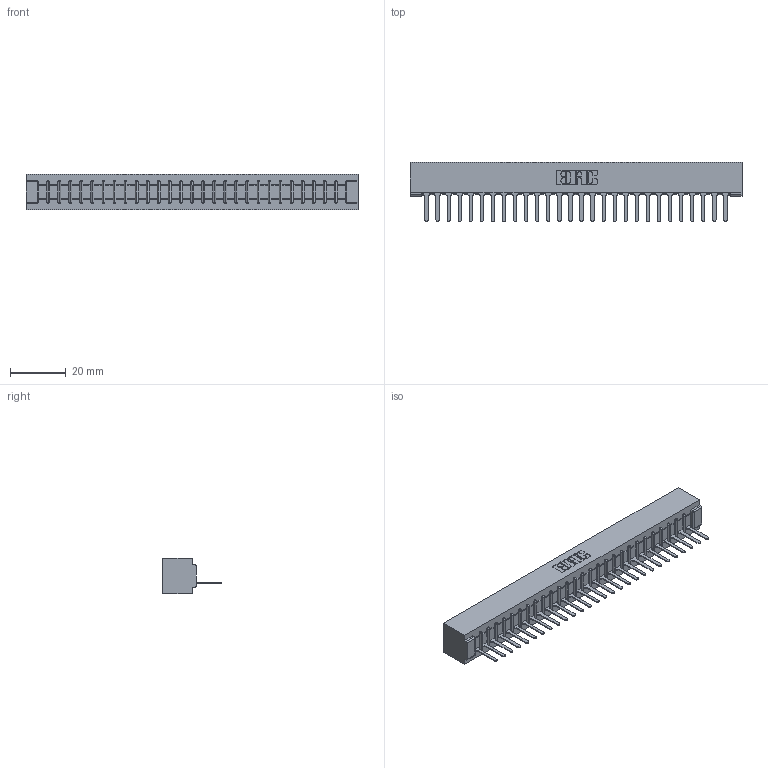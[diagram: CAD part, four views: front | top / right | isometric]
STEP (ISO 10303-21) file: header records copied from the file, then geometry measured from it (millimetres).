
FILE_DESCRIPTION (( 'STEP AP203' ), '1' );
FILE_NAME ('357-028-427-101.STEP', '2020-10-01T20:28:08', ( '' ), ( '' ), 'SwSTEP 2.0', 'SolidWorks 2020', '' );
FILE_SCHEMA (( 'CONFIG_CONTROL_DESIGN' ));
Length unit declared in the file: inch
Products named in the file (3): 307-290-001_527; 307 Part_No Mounting Lugs; 357-028-427-101
Assembly tree (29 placements, depth 2):
  357-028-427-101
    307 Part_No Mounting Lugs
    307-290-001_527  x28
Bounding box: 118.82 x 21.11 x 12.7 mm (x, y, z)
Volume: 12782.6 mm3; surface area: 13606.4 mm2
Topology: 29 solids, 29 shells, 1707 faces, 4835 edges, 3106 vertices
Faces by surface type: plane 1102, cylinder 547, sphere 58
Entity records: 25420 total; most frequent: CARTESIAN_POINT 4276, ORIENTED_EDGE 4262, DIRECTION 4165, EDGE_CURVE 2131, LINE 1631, VECTOR 1631, VERTEX_POINT 1378, AXIS2_PLACEMENT_3D 1267
